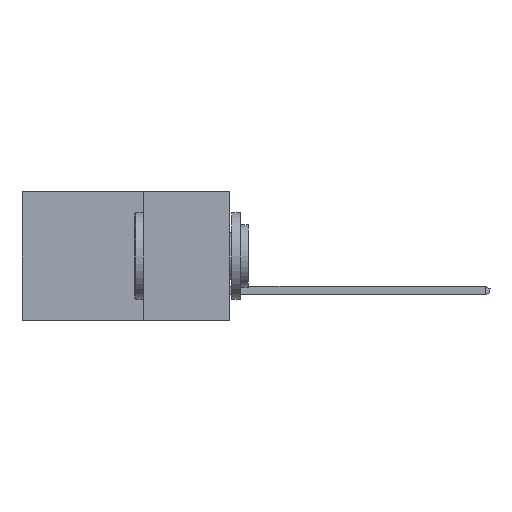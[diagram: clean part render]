
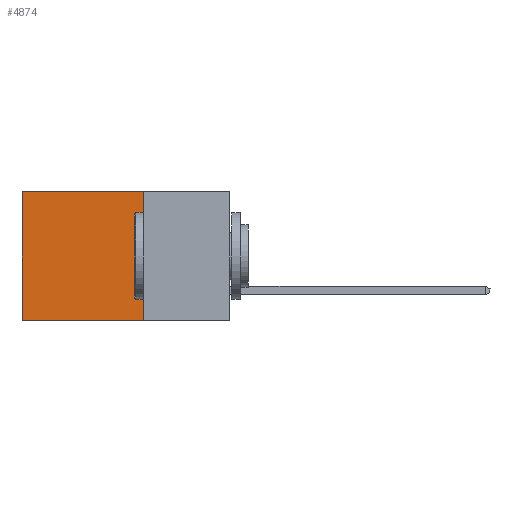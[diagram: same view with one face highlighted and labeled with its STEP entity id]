
A CAD part, left-side view. The second image highlights one B-rep face of the part: STEP entity #4874.
In plain terms, the highlighted planar face has unit normal (-1, 0, 0).
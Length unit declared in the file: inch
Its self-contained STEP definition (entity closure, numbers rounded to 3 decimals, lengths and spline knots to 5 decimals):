
#267 = DIRECTION ( 'NONE',  ( 1., 0., 0. ) ) ;
#315 = LINE ( 'NONE', #15361, #4334 ) ;
#1073 = EDGE_CURVE ( 'NONE', #13601, #14054, #315, .T. ) ;
#2058 = LINE ( 'NONE', #12922, #12192 ) ;
#3084 = EDGE_CURVE ( 'NONE', #12719, #13601, #15857, .T. ) ;
#4034 = CARTESIAN_POINT ( 'NONE',  ( 0.2615, 0.6, 0. ) ) ;
#4334 = VECTOR ( 'NONE', #11129, 39.37008 ) ;
#4721 = EDGE_LOOP ( 'NONE', ( #17400, #7489, #11586, #6686 ) ) ;
#4874 = ADVANCED_FACE ( 'NONE', ( #7184 ), #8435, .F. ) ;
#5437 = CARTESIAN_POINT ( 'NONE',  ( 0.2615, 0.25, 0. ) ) ;
#6450 = CARTESIAN_POINT ( 'NONE',  ( 0.2615, 0.25, -0.37 ) ) ;
#6555 = CARTESIAN_POINT ( 'NONE',  ( 0.2615, 0.25, -0.37 ) ) ;
#6621 = DIRECTION ( 'NONE',  ( 0., 1., 0. ) ) ;
#6686 = ORIENTED_EDGE ( 'NONE', *, *, #3084, .T. ) ;
#6714 = LINE ( 'NONE', #6450, #16621 ) ;
#6877 = EDGE_CURVE ( 'NONE', #7590, #14054, #6714, .T. ) ;
#7184 = FACE_OUTER_BOUND ( 'NONE', #4721, .T. ) ;
#7489 = ORIENTED_EDGE ( 'NONE', *, *, #6877, .F. ) ;
#7590 = VERTEX_POINT ( 'NONE', #6555 ) ;
#8351 = CARTESIAN_POINT ( 'NONE',  ( 0.2615, 0.25, -0.37 ) ) ;
#8435 = PLANE ( 'NONE',  #14828 ) ;
#9106 = EDGE_CURVE ( 'NONE', #12719, #7590, #2058, .T. ) ;
#10830 = DIRECTION ( 'NONE',  ( 0., 1., 0. ) ) ;
#11129 = DIRECTION ( 'NONE',  ( 0., 0., -1. ) ) ;
#11586 = ORIENTED_EDGE ( 'NONE', *, *, #9106, .F. ) ;
#12192 = VECTOR ( 'NONE', #13999, 39.37008 ) ;
#12550 = DIRECTION ( 'NONE',  ( 0., 0., -1. ) ) ;
#12719 = VERTEX_POINT ( 'NONE', #13293 ) ;
#12922 = CARTESIAN_POINT ( 'NONE',  ( 0.2615, 0.25, -0.37 ) ) ;
#13110 = CARTESIAN_POINT ( 'NONE',  ( 0.2615, 0.6, -0.37 ) ) ;
#13169 = VECTOR ( 'NONE', #10830, 39.37008 ) ;
#13293 = CARTESIAN_POINT ( 'NONE',  ( 0.2615, 0.25, 0. ) ) ;
#13601 = VERTEX_POINT ( 'NONE', #4034 ) ;
#13999 = DIRECTION ( 'NONE',  ( 0., 0., -1. ) ) ;
#14054 = VERTEX_POINT ( 'NONE', #13110 ) ;
#14828 = AXIS2_PLACEMENT_3D ( 'NONE', #8351, #267, #12550 ) ;
#15361 = CARTESIAN_POINT ( 'NONE',  ( 0.2615, 0.6, -0.37 ) ) ;
#15857 = LINE ( 'NONE', #5437, #13169 ) ;
#16621 = VECTOR ( 'NONE', #6621, 39.37008 ) ;
#17400 = ORIENTED_EDGE ( 'NONE', *, *, #1073, .T. ) ;
